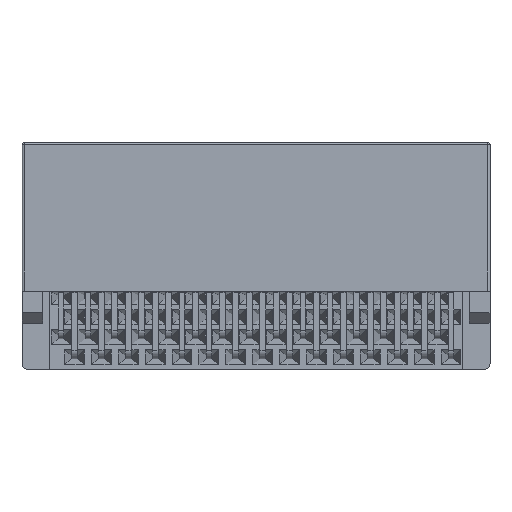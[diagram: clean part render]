
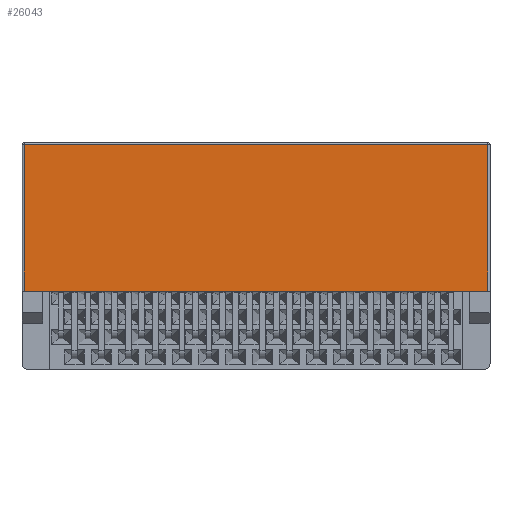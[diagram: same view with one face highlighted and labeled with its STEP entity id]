
A CAD part, top view. The second image highlights one B-rep face of the part: STEP entity #26043.
In plain terms, the highlighted planar face has unit normal (0, 0, 1).
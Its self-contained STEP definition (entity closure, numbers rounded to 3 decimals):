
#1175 = VECTOR ( 'NONE', #33773, 1000. ) ;
#1260 = CARTESIAN_POINT ( 'NONE',  ( 44., 1.5, 0. ) ) ;
#2610 = VECTOR ( 'NONE', #15715, 1000. ) ;
#3291 = CARTESIAN_POINT ( 'NONE',  ( 44., 15.5, 0. ) ) ;
#3647 = VERTEX_POINT ( 'NONE', #29706 ) ;
#4124 = VERTEX_POINT ( 'NONE', #1260 ) ;
#4244 = EDGE_CURVE ( 'NONE', #4124, #4535, #33637, .T. ) ;
#4535 = VERTEX_POINT ( 'NONE', #29812 ) ;
#5415 = AXIS2_PLACEMENT_3D ( 'NONE', #35413, #9314, #18060 ) ;
#6873 = EDGE_LOOP ( 'NONE', ( #28072, #21329, #29006, #37328 ) ) ;
#9314 = DIRECTION ( 'NONE',  ( 0., 0., -1. ) ) ;
#9774 = DIRECTION ( 'NONE',  ( 0., 1., 0. ) ) ;
#12170 = FACE_OUTER_BOUND ( 'NONE', #6873, .T. ) ;
#15715 = DIRECTION ( 'NONE',  ( -1., 0., 0. ) ) ;
#18060 = DIRECTION ( 'NONE',  ( -1., 0., 0. ) ) ;
#19162 = DIRECTION ( 'NONE',  ( -1., 0., 0. ) ) ;
#21234 = VERTEX_POINT ( 'NONE', #25265 ) ;
#21329 = ORIENTED_EDGE ( 'NONE', *, *, #34063, .T. ) ;
#21815 = CARTESIAN_POINT ( 'NONE',  ( 0., 15.3, 0. ) ) ;
#22166 = LINE ( 'NONE', #33595, #1175 ) ;
#22211 = CARTESIAN_POINT ( 'NONE',  ( 44.2, 1.5, 0. ) ) ;
#22801 = EDGE_CURVE ( 'NONE', #3647, #21234, #24300, .T. ) ;
#23799 = PLANE ( 'NONE',  #5415 ) ;
#24300 = LINE ( 'NONE', #21815, #2610 ) ;
#25265 = CARTESIAN_POINT ( 'NONE',  ( 0.2, 15.3, 0. ) ) ;
#26043 = ADVANCED_FACE ( 'NONE', ( #12170 ), #23799, .F. ) ;
#28072 = ORIENTED_EDGE ( 'NONE', *, *, #4244, .F. ) ;
#29006 = ORIENTED_EDGE ( 'NONE', *, *, #22801, .T. ) ;
#29706 = CARTESIAN_POINT ( 'NONE',  ( 44., 15.3, 0. ) ) ;
#29812 = CARTESIAN_POINT ( 'NONE',  ( 0.2, 1.5, 0. ) ) ;
#30288 = VECTOR ( 'NONE', #9774, 1000. ) ;
#31234 = VECTOR ( 'NONE', #19162, 1000. ) ;
#32433 = LINE ( 'NONE', #3291, #30288 ) ;
#32513 = EDGE_CURVE ( 'NONE', #21234, #4535, #22166, .T. ) ;
#33595 = CARTESIAN_POINT ( 'NONE',  ( 0.2, 15.5, 0. ) ) ;
#33637 = LINE ( 'NONE', #22211, #31234 ) ;
#33773 = DIRECTION ( 'NONE',  ( 0., -1., 0. ) ) ;
#34063 = EDGE_CURVE ( 'NONE', #4124, #3647, #32433, .T. ) ;
#35413 = CARTESIAN_POINT ( 'NONE',  ( 0., 15.5, 0. ) ) ;
#37328 = ORIENTED_EDGE ( 'NONE', *, *, #32513, .T. ) ;
